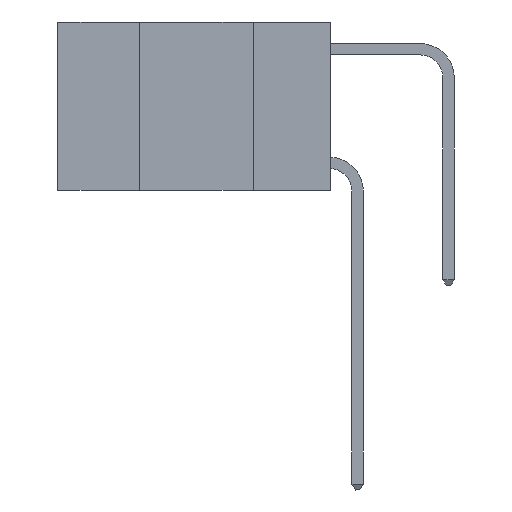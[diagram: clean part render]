
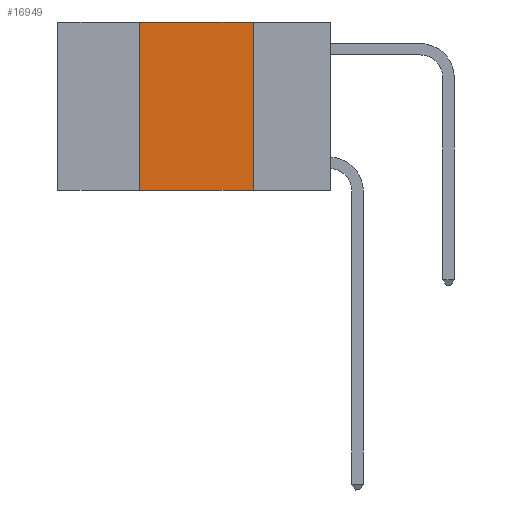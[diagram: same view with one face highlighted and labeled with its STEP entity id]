
A CAD part, left-side view. The second image highlights one B-rep face of the part: STEP entity #16949.
In plain terms, the highlighted planar face has unit normal (-1, 0, 0).
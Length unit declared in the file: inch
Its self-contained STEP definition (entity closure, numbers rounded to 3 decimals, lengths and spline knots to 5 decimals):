
#223 = VERTEX_POINT ( 'NONE', #30976 ) ;
#732 = VECTOR ( 'NONE', #25627, 39.37008 ) ;
#1860 = CARTESIAN_POINT ( 'NONE',  ( 0., 0.42, 0. ) ) ;
#2566 = EDGE_CURVE ( 'NONE', #23308, #15565, #20297, .T. ) ;
#3586 = CARTESIAN_POINT ( 'NONE',  ( 0., 0.17, 0. ) ) ;
#3921 = VERTEX_POINT ( 'NONE', #18094 ) ;
#4646 = EDGE_CURVE ( 'NONE', #3921, #223, #20564, .T. ) ;
#8059 = DIRECTION ( 'NONE',  ( 0., 0., -1. ) ) ;
#9170 = ORIENTED_EDGE ( 'NONE', *, *, #21679, .F. ) ;
#9516 = VECTOR ( 'NONE', #8059, 39.37008 ) ;
#10475 = EDGE_LOOP ( 'NONE', ( #26856, #29333, #9170, #30549 ) ) ;
#10719 = DIRECTION ( 'NONE',  ( 1., 0., 0. ) ) ;
#12446 = VECTOR ( 'NONE', #30519, 39.37008 ) ;
#14747 = AXIS2_PLACEMENT_3D ( 'NONE', #16040, #10719, #21322 ) ;
#14765 = CARTESIAN_POINT ( 'NONE',  ( 0., 0.6, 0. ) ) ;
#15540 = CARTESIAN_POINT ( 'NONE',  ( 0., 0.6, -0.37 ) ) ;
#15565 = VERTEX_POINT ( 'NONE', #3586 ) ;
#16034 = VECTOR ( 'NONE', #23250, 39.37008 ) ;
#16040 = CARTESIAN_POINT ( 'NONE',  ( 0., 0.6, 0. ) ) ;
#16053 = FACE_OUTER_BOUND ( 'NONE', #10475, .T. ) ;
#16466 = LINE ( 'NONE', #1860, #732 ) ;
#16674 = CARTESIAN_POINT ( 'NONE',  ( 0., 0.42, 0. ) ) ;
#16949 = ADVANCED_FACE ( 'NONE', ( #16053 ), #18674, .F. ) ;
#18094 = CARTESIAN_POINT ( 'NONE',  ( 0., 0.42, -0.37 ) ) ;
#18674 = PLANE ( 'NONE',  #14747 ) ;
#20297 = LINE ( 'NONE', #14765, #12446 ) ;
#20564 = LINE ( 'NONE', #15540, #16034 ) ;
#20684 = EDGE_CURVE ( 'NONE', #15565, #223, #23524, .T. ) ;
#21322 = DIRECTION ( 'NONE',  ( 0., 0., -1. ) ) ;
#21679 = EDGE_CURVE ( 'NONE', #3921, #23308, #16466, .T. ) ;
#23250 = DIRECTION ( 'NONE',  ( 0., -1., 0. ) ) ;
#23308 = VERTEX_POINT ( 'NONE', #16674 ) ;
#23524 = LINE ( 'NONE', #26482, #9516 ) ;
#25627 = DIRECTION ( 'NONE',  ( 0., 0., 1. ) ) ;
#26482 = CARTESIAN_POINT ( 'NONE',  ( 0., 0.17, 0. ) ) ;
#26856 = ORIENTED_EDGE ( 'NONE', *, *, #20684, .F. ) ;
#29333 = ORIENTED_EDGE ( 'NONE', *, *, #2566, .F. ) ;
#30519 = DIRECTION ( 'NONE',  ( 0., -1., 0. ) ) ;
#30549 = ORIENTED_EDGE ( 'NONE', *, *, #4646, .T. ) ;
#30976 = CARTESIAN_POINT ( 'NONE',  ( 0., 0.17, -0.37 ) ) ;
